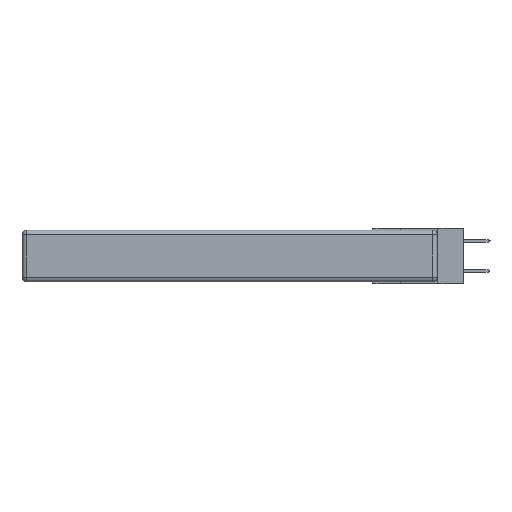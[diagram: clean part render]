
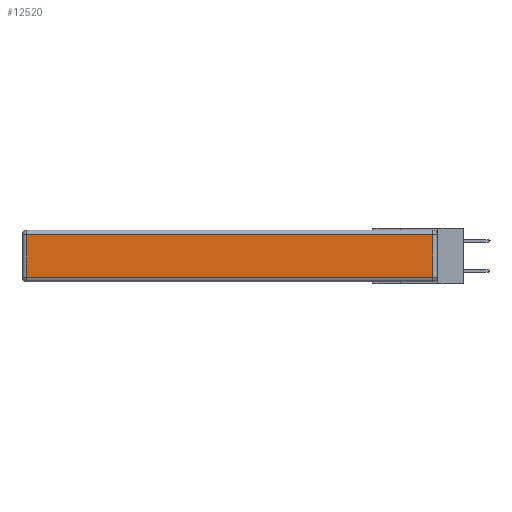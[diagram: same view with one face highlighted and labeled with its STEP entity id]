
A CAD part, left-side view. The second image highlights one B-rep face of the part: STEP entity #12520.
In plain terms, the highlighted planar face has unit normal (-1, 0, 0).
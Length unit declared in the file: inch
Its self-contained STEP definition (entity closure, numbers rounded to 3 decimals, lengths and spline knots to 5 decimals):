
#22 = VERTEX_POINT ( 'NONE', #7472 ) ;
#105 = DIRECTION ( 'NONE',  ( -1., 0., 0. ) ) ;
#137 = DIRECTION ( 'NONE',  ( 0., 0., 1. ) ) ;
#582 = ORIENTED_EDGE ( 'NONE', *, *, #9840, .T. ) ;
#648 = CARTESIAN_POINT ( 'NONE',  ( 0., 2.72, -0.343 ) ) ;
#1225 = VERTEX_POINT ( 'NONE', #6864 ) ;
#1377 = CARTESIAN_POINT ( 'NONE',  ( 0., 2.75, -0.03 ) ) ;
#1600 = VECTOR ( 'NONE', #137, 39.37008 ) ;
#2474 = DIRECTION ( 'NONE',  ( 0., -1., 0. ) ) ;
#2774 = EDGE_CURVE ( 'NONE', #11878, #8684, #3212, .T. ) ;
#2851 = LINE ( 'NONE', #4099, #1600 ) ;
#3212 = LINE ( 'NONE', #8382, #8213 ) ;
#4026 = CARTESIAN_POINT ( 'NONE',  ( 0., 0., -0.343 ) ) ;
#4099 = CARTESIAN_POINT ( 'NONE',  ( 0., 0.03, -0.343 ) ) ;
#4205 = AXIS2_PLACEMENT_3D ( 'NONE', #4026, #105, #9172 ) ;
#4642 = DIRECTION ( 'NONE',  ( 0., 1., 0. ) ) ;
#5435 = EDGE_CURVE ( 'NONE', #1225, #22, #8019, .T. ) ;
#6255 = VECTOR ( 'NONE', #9648, 39.37008 ) ;
#6864 = CARTESIAN_POINT ( 'NONE',  ( 0., 0.03, -0.03 ) ) ;
#7472 = CARTESIAN_POINT ( 'NONE',  ( 0., 2.72, -0.03 ) ) ;
#8019 = LINE ( 'NONE', #1377, #12109 ) ;
#8213 = VECTOR ( 'NONE', #2474, 39.37008 ) ;
#8382 = CARTESIAN_POINT ( 'NONE',  ( 0., 0., -0.313 ) ) ;
#8684 = VERTEX_POINT ( 'NONE', #10084 ) ;
#8744 = ORIENTED_EDGE ( 'NONE', *, *, #5435, .T. ) ;
#9172 = DIRECTION ( 'NONE',  ( 0., 0., 1. ) ) ;
#9215 = PLANE ( 'NONE',  #4205 ) ;
#9648 = DIRECTION ( 'NONE',  ( 0., 0., -1. ) ) ;
#9840 = EDGE_CURVE ( 'NONE', #8684, #1225, #2851, .T. ) ;
#10084 = CARTESIAN_POINT ( 'NONE',  ( 0., 0.03, -0.313 ) ) ;
#10450 = CARTESIAN_POINT ( 'NONE',  ( 0., 2.72, -0.313 ) ) ;
#10676 = LINE ( 'NONE', #648, #6255 ) ;
#11149 = ORIENTED_EDGE ( 'NONE', *, *, #11236, .T. ) ;
#11215 = ORIENTED_EDGE ( 'NONE', *, *, #2774, .T. ) ;
#11236 = EDGE_CURVE ( 'NONE', #22, #11878, #10676, .T. ) ;
#11260 = FACE_OUTER_BOUND ( 'NONE', #12756, .T. ) ;
#11878 = VERTEX_POINT ( 'NONE', #10450 ) ;
#12109 = VECTOR ( 'NONE', #4642, 39.37008 ) ;
#12520 = ADVANCED_FACE ( 'NONE', ( #11260 ), #9215, .T. ) ;
#12756 = EDGE_LOOP ( 'NONE', ( #11215, #582, #8744, #11149 ) ) ;
